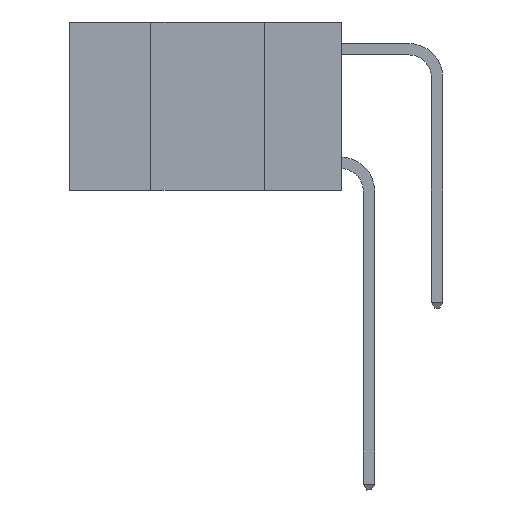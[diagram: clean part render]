
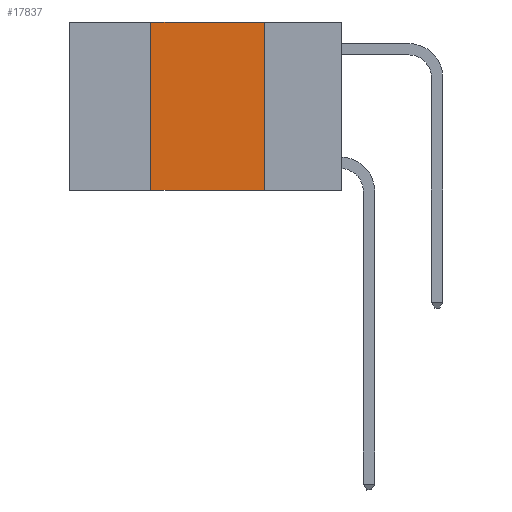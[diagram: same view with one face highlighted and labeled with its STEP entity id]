
A CAD part, left-side view. The second image highlights one B-rep face of the part: STEP entity #17837.
In plain terms, the highlighted planar face has unit normal (-1, 0, 0).
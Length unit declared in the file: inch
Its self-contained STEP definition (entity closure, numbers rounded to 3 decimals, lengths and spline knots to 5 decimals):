
#455 = DIRECTION ( 'NONE',  ( 0., 0., -1. ) ) ;
#1132 = CARTESIAN_POINT ( 'NONE',  ( 0., 0.6, -0.37 ) ) ;
#2344 = VECTOR ( 'NONE', #21347, 39.37008 ) ;
#2873 = CARTESIAN_POINT ( 'NONE',  ( 0., 0.42, -0.37 ) ) ;
#3623 = EDGE_CURVE ( 'NONE', #13597, #20518, #8018, .T. ) ;
#5931 = CARTESIAN_POINT ( 'NONE',  ( 0., 0.6, 0. ) ) ;
#5993 = PLANE ( 'NONE',  #18707 ) ;
#6334 = FACE_OUTER_BOUND ( 'NONE', #17840, .T. ) ;
#7170 = CARTESIAN_POINT ( 'NONE',  ( 0., 0.42, 0. ) ) ;
#8018 = LINE ( 'NONE', #1132, #10963 ) ;
#8092 = VECTOR ( 'NONE', #13131, 39.37008 ) ;
#9808 = EDGE_CURVE ( 'NONE', #13597, #22644, #10716, .T. ) ;
#10518 = EDGE_CURVE ( 'NONE', #18236, #20518, #16922, .T. ) ;
#10716 = LINE ( 'NONE', #7170, #2344 ) ;
#10963 = VECTOR ( 'NONE', #13252, 39.37008 ) ;
#11047 = CARTESIAN_POINT ( 'NONE',  ( 0., 0.17, 0. ) ) ;
#13131 = DIRECTION ( 'NONE',  ( 0., -1., 0. ) ) ;
#13252 = DIRECTION ( 'NONE',  ( 0., -1., 0. ) ) ;
#13597 = VERTEX_POINT ( 'NONE', #2873 ) ;
#13797 = ORIENTED_EDGE ( 'NONE', *, *, #15575, .F. ) ;
#14437 = ORIENTED_EDGE ( 'NONE', *, *, #9808, .F. ) ;
#14645 = CARTESIAN_POINT ( 'NONE',  ( 0., 0.42, 0. ) ) ;
#14782 = CARTESIAN_POINT ( 'NONE',  ( 0., 0.17, -0.37 ) ) ;
#15176 = CARTESIAN_POINT ( 'NONE',  ( 0., 0.17, 0. ) ) ;
#15575 = EDGE_CURVE ( 'NONE', #22644, #18236, #22105, .T. ) ;
#16922 = LINE ( 'NONE', #15176, #21642 ) ;
#16951 = CARTESIAN_POINT ( 'NONE',  ( 0., 0.6, 0. ) ) ;
#17837 = ADVANCED_FACE ( 'NONE', ( #6334 ), #5993, .F. ) ;
#17840 = EDGE_LOOP ( 'NONE', ( #22532, #13797, #14437, #19568 ) ) ;
#18236 = VERTEX_POINT ( 'NONE', #11047 ) ;
#18700 = DIRECTION ( 'NONE',  ( 1., 0., 0. ) ) ;
#18707 = AXIS2_PLACEMENT_3D ( 'NONE', #16951, #18700, #22400 ) ;
#19568 = ORIENTED_EDGE ( 'NONE', *, *, #3623, .T. ) ;
#20518 = VERTEX_POINT ( 'NONE', #14782 ) ;
#21347 = DIRECTION ( 'NONE',  ( 0., 0., 1. ) ) ;
#21642 = VECTOR ( 'NONE', #455, 39.37008 ) ;
#22105 = LINE ( 'NONE', #5931, #8092 ) ;
#22400 = DIRECTION ( 'NONE',  ( 0., 0., -1. ) ) ;
#22532 = ORIENTED_EDGE ( 'NONE', *, *, #10518, .F. ) ;
#22644 = VERTEX_POINT ( 'NONE', #14645 ) ;
